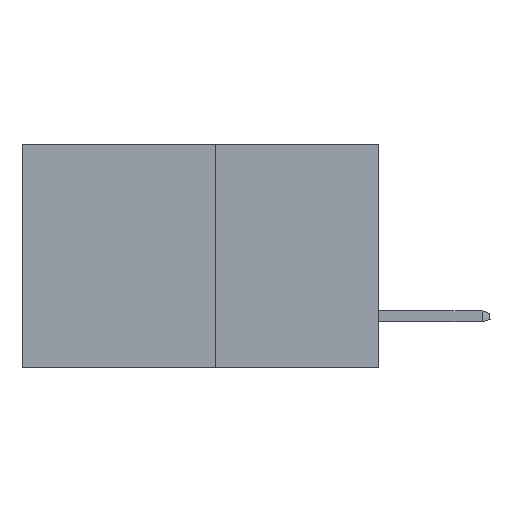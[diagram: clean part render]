
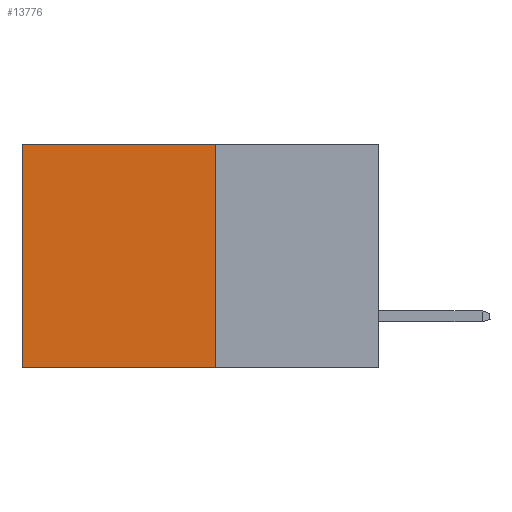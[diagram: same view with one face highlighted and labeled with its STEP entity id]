
A CAD part, left-side view. The second image highlights one B-rep face of the part: STEP entity #13776.
In plain terms, the highlighted planar face has unit normal (-1, 0, 0).
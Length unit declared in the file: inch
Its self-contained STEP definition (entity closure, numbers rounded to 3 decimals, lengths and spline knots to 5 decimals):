
#37 = EDGE_CURVE ( 'NONE', #447, #10387, #8948, .T. ) ;
#447 = VERTEX_POINT ( 'NONE', #514 ) ;
#514 = CARTESIAN_POINT ( 'NONE',  ( 0.277, 0.27, 0. ) ) ;
#614 = CARTESIAN_POINT ( 'NONE',  ( 0.277, 0.59, -0.37 ) ) ;
#883 = ORIENTED_EDGE ( 'NONE', *, *, #3088, .T. ) ;
#926 = ORIENTED_EDGE ( 'NONE', *, *, #11071, .F. ) ;
#999 = EDGE_CURVE ( 'NONE', #447, #10103, #4302, .T. ) ;
#1083 = ORIENTED_EDGE ( 'NONE', *, *, #999, .F. ) ;
#1245 = CARTESIAN_POINT ( 'NONE',  ( 0.277, 0.59, 0. ) ) ;
#1540 = ORIENTED_EDGE ( 'NONE', *, *, #37, .T. ) ;
#3088 = EDGE_CURVE ( 'NONE', #10387, #8159, #17434, .T. ) ;
#3120 = CARTESIAN_POINT ( 'NONE',  ( 0.277, 0.27, -0.37 ) ) ;
#3124 = EDGE_LOOP ( 'NONE', ( #883, #926, #1083, #1540 ) ) ;
#3407 = VECTOR ( 'NONE', #4660, 39.37008 ) ;
#4302 = LINE ( 'NONE', #3120, #3407 ) ;
#4660 = DIRECTION ( 'NONE',  ( 0., 0., -1. ) ) ;
#5138 = AXIS2_PLACEMENT_3D ( 'NONE', #8187, #16483, #8249 ) ;
#8159 = VERTEX_POINT ( 'NONE', #614 ) ;
#8187 = CARTESIAN_POINT ( 'NONE',  ( 0.277, 0.27, -0.37 ) ) ;
#8249 = DIRECTION ( 'NONE',  ( 0., 0., -1. ) ) ;
#8441 = DIRECTION ( 'NONE',  ( 0., 1., 0. ) ) ;
#8948 = LINE ( 'NONE', #16759, #12199 ) ;
#9333 = LINE ( 'NONE', #18070, #12126 ) ;
#10103 = VERTEX_POINT ( 'NONE', #13003 ) ;
#10105 = FACE_OUTER_BOUND ( 'NONE', #3124, .T. ) ;
#10387 = VERTEX_POINT ( 'NONE', #1245 ) ;
#11071 = EDGE_CURVE ( 'NONE', #10103, #8159, #9333, .T. ) ;
#11793 = DIRECTION ( 'NONE',  ( 0., 1., 0. ) ) ;
#12126 = VECTOR ( 'NONE', #8441, 39.37008 ) ;
#12199 = VECTOR ( 'NONE', #11793, 39.37008 ) ;
#13003 = CARTESIAN_POINT ( 'NONE',  ( 0.277, 0.27, -0.37 ) ) ;
#13748 = PLANE ( 'NONE',  #5138 ) ;
#13776 = ADVANCED_FACE ( 'NONE', ( #10105 ), #13748, .F. ) ;
#13794 = VECTOR ( 'NONE', #17674, 39.37008 ) ;
#14914 = CARTESIAN_POINT ( 'NONE',  ( 0.277, 0.59, -0.37 ) ) ;
#16483 = DIRECTION ( 'NONE',  ( 1., 0., 0. ) ) ;
#16759 = CARTESIAN_POINT ( 'NONE',  ( 0.277, 0.27, 0. ) ) ;
#17434 = LINE ( 'NONE', #14914, #13794 ) ;
#17674 = DIRECTION ( 'NONE',  ( 0., 0., -1. ) ) ;
#18070 = CARTESIAN_POINT ( 'NONE',  ( 0.277, 0.27, -0.37 ) ) ;
